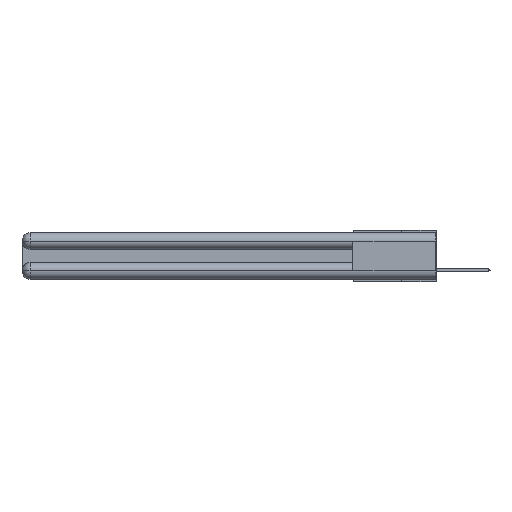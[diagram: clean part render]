
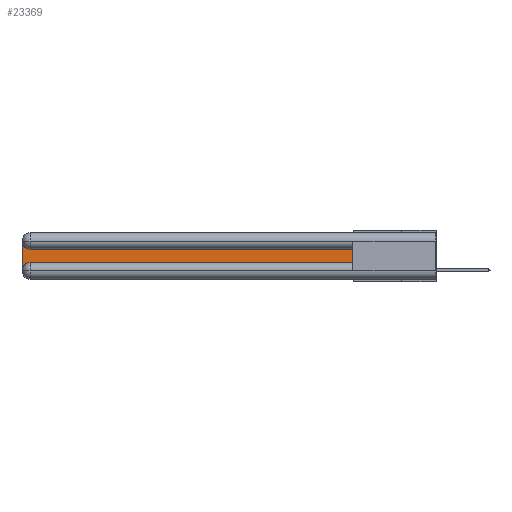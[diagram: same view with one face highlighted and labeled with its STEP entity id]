
A CAD part, left-side view. The second image highlights one B-rep face of the part: STEP entity #23369.
In plain terms, the highlighted planar face has unit normal (-1, 0, 0).
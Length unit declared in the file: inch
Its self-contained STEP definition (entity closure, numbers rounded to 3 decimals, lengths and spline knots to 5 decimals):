
#67 = EDGE_CURVE ( 'NONE', #3601, #1177, #1945, .T. ) ;
#1177 = VERTEX_POINT ( 'NONE', #7526 ) ;
#1945 = LINE ( 'NONE', #10588, #21542 ) ;
#2049 = DIRECTION ( 'NONE',  ( 1., 0., 0. ) ) ;
#2244 = ORIENTED_EDGE ( 'NONE', *, *, #23368, .T. ) ;
#2636 = VECTOR ( 'NONE', #26724, 39.37008 ) ;
#2682 = VECTOR ( 'NONE', #20251, 39.37008 ) ;
#3358 = VERTEX_POINT ( 'NONE', #22872 ) ;
#3396 = CARTESIAN_POINT ( 'NONE',  ( 0.075, 2.94, -0.2175 ) ) ;
#3543 = CARTESIAN_POINT ( 'NONE',  ( 0.075, 3., -0.2775 ) ) ;
#3601 = VERTEX_POINT ( 'NONE', #27982 ) ;
#4282 = CARTESIAN_POINT ( 'NONE',  ( 0.075, 0.6, -0.2175 ) ) ;
#4515 = EDGE_LOOP ( 'NONE', ( #24413, #2244, #19138, #18289, #17150, #19059 ) ) ;
#5393 = AXIS2_PLACEMENT_3D ( 'NONE', #19730, #8680, #22283 ) ;
#5813 = EDGE_CURVE ( 'NONE', #3358, #7415, #20544, .T. ) ;
#7415 = VERTEX_POINT ( 'NONE', #3543 ) ;
#7465 = AXIS2_PLACEMENT_3D ( 'NONE', #9283, #24948, #27473 ) ;
#7526 = CARTESIAN_POINT ( 'NONE',  ( 0.075, 2.94, -0.1225 ) ) ;
#7740 = EDGE_CURVE ( 'NONE', #12142, #24236, #8562, .T. ) ;
#8340 = DIRECTION ( 'NONE',  ( 0., 0., -1. ) ) ;
#8562 = LINE ( 'NONE', #4282, #2636 ) ;
#8680 = DIRECTION ( 'NONE',  ( 1., 0., 0. ) ) ;
#9283 = CARTESIAN_POINT ( 'NONE',  ( 0.075, 2.94, -0.2775 ) ) ;
#10070 = VECTOR ( 'NONE', #8340, 39.37008 ) ;
#10588 = CARTESIAN_POINT ( 'NONE',  ( 0.075, 0.6, -0.1225 ) ) ;
#10837 = PLANE ( 'NONE',  #25442 ) ;
#11033 = DIRECTION ( 'NONE',  ( 0., 0., -1. ) ) ;
#11261 = CARTESIAN_POINT ( 'NONE',  ( 0.075, 0.6, -0.2175 ) ) ;
#11674 = EDGE_CURVE ( 'NONE', #7415, #12142, #17056, .T. ) ;
#12142 = VERTEX_POINT ( 'NONE', #3396 ) ;
#12583 = CIRCLE ( 'NONE', #5393, 0.06 ) ;
#12638 = CARTESIAN_POINT ( 'NONE',  ( 0.075, 3., -0.2175 ) ) ;
#17056 = CIRCLE ( 'NONE', #7465, 0.06 ) ;
#17150 = ORIENTED_EDGE ( 'NONE', *, *, #7740, .T. ) ;
#18289 = ORIENTED_EDGE ( 'NONE', *, *, #11674, .T. ) ;
#19059 = ORIENTED_EDGE ( 'NONE', *, *, #24632, .T. ) ;
#19138 = ORIENTED_EDGE ( 'NONE', *, *, #5813, .T. ) ;
#19393 = DIRECTION ( 'NONE',  ( 0., 1., 0. ) ) ;
#19730 = CARTESIAN_POINT ( 'NONE',  ( 0.075, 2.94, -0.0625 ) ) ;
#20251 = DIRECTION ( 'NONE',  ( 0., 0., 1. ) ) ;
#20544 = LINE ( 'NONE', #12638, #10070 ) ;
#20660 = CARTESIAN_POINT ( 'NONE',  ( 0.075, 0.6, -0.2175 ) ) ;
#21542 = VECTOR ( 'NONE', #19393, 39.37008 ) ;
#22283 = DIRECTION ( 'NONE',  ( 0., 0., -1. ) ) ;
#22872 = CARTESIAN_POINT ( 'NONE',  ( 0.075, 3., -0.0625 ) ) ;
#23368 = EDGE_CURVE ( 'NONE', #1177, #3358, #12583, .T. ) ;
#23369 = ADVANCED_FACE ( 'NONE', ( #23426 ), #10837, .F. ) ;
#23426 = FACE_OUTER_BOUND ( 'NONE', #4515, .T. ) ;
#24236 = VERTEX_POINT ( 'NONE', #20660 ) ;
#24413 = ORIENTED_EDGE ( 'NONE', *, *, #67, .T. ) ;
#24632 = EDGE_CURVE ( 'NONE', #24236, #3601, #26865, .T. ) ;
#24948 = DIRECTION ( 'NONE',  ( 1., 0., 0. ) ) ;
#25442 = AXIS2_PLACEMENT_3D ( 'NONE', #28863, #2049, #11033 ) ;
#26724 = DIRECTION ( 'NONE',  ( 0., -1., 0. ) ) ;
#26865 = LINE ( 'NONE', #11261, #2682 ) ;
#27473 = DIRECTION ( 'NONE',  ( 0., 0., -1. ) ) ;
#27982 = CARTESIAN_POINT ( 'NONE',  ( 0.075, 0.6, -0.1225 ) ) ;
#28863 = CARTESIAN_POINT ( 'NONE',  ( 0.075, 3., -0.1225 ) ) ;
